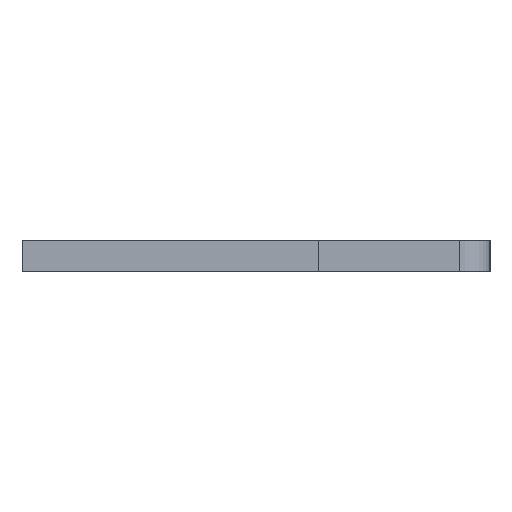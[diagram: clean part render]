
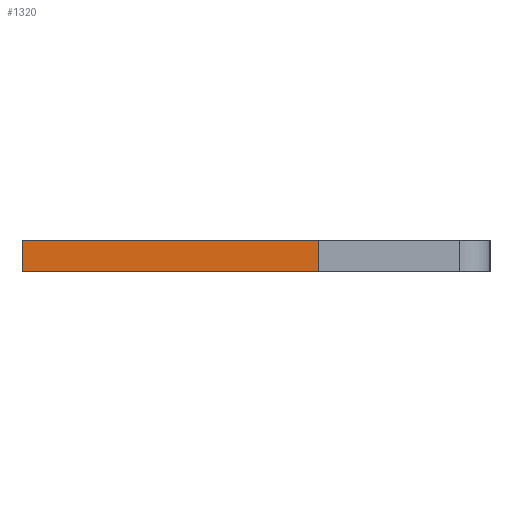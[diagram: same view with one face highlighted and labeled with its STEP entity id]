
A CAD part, left-side view. The second image highlights one B-rep face of the part: STEP entity #1320.
In plain terms, the highlighted face is planar.
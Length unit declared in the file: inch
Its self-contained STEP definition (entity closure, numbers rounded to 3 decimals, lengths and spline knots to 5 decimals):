
#26 = DIRECTION ( 'NONE',  ( -1., 0., 0. ) ) ;
#73 = EDGE_LOOP ( 'NONE', ( #1088, #316, #268, #369 ) ) ;
#86 = VECTOR ( 'NONE', #849, 39.37008 ) ;
#99 = CARTESIAN_POINT ( 'NONE',  ( 0.01, 0.15, -0.04 ) ) ;
#104 = CARTESIAN_POINT ( 'NONE',  ( 0.01, -0.04, -0.04 ) ) ;
#106 = EDGE_CURVE ( 'NONE', #1001, #947, #1057, .T. ) ;
#175 = CARTESIAN_POINT ( 'NONE',  ( -0.01, -0.04, -0.04 ) ) ;
#210 = DIRECTION ( 'NONE',  ( -1., 0., 0. ) ) ;
#268 = ORIENTED_EDGE ( 'NONE', *, *, #494, .F. ) ;
#316 = ORIENTED_EDGE ( 'NONE', *, *, #1293, .F. ) ;
#329 = CARTESIAN_POINT ( 'NONE',  ( 0.01, 0.15, -0.04 ) ) ;
#353 = VECTOR ( 'NONE', #26, 39.37008 ) ;
#369 = ORIENTED_EDGE ( 'NONE', *, *, #448, .T. ) ;
#383 = VECTOR ( 'NONE', #591, 39.37008 ) ;
#416 = CARTESIAN_POINT ( 'NONE',  ( 0.01, 0.15, -0.04 ) ) ;
#446 = FACE_OUTER_BOUND ( 'NONE', #73, .T. ) ;
#448 = EDGE_CURVE ( 'NONE', #934, #1001, #1287, .T. ) ;
#465 = CARTESIAN_POINT ( 'NONE',  ( 0.01, 0.15, -0.04 ) ) ;
#494 = EDGE_CURVE ( 'NONE', #934, #701, #1094, .T. ) ;
#528 = DIRECTION ( 'NONE',  ( 1., 0., 0. ) ) ;
#591 = DIRECTION ( 'NONE',  ( 0., 1., 0. ) ) ;
#598 = AXIS2_PLACEMENT_3D ( 'NONE', #329, #1306, #528 ) ;
#628 = VECTOR ( 'NONE', #210, 39.37008 ) ;
#642 = PLANE ( 'NONE',  #598 ) ;
#701 = VERTEX_POINT ( 'NONE', #465 ) ;
#794 = CARTESIAN_POINT ( 'NONE',  ( -0.01, 0.15, -0.04 ) ) ;
#849 = DIRECTION ( 'NONE',  ( 0., 1., 0. ) ) ;
#934 = VERTEX_POINT ( 'NONE', #1224 ) ;
#947 = VERTEX_POINT ( 'NONE', #794 ) ;
#1001 = VERTEX_POINT ( 'NONE', #175 ) ;
#1057 = LINE ( 'NONE', #1135, #383 ) ;
#1088 = ORIENTED_EDGE ( 'NONE', *, *, #106, .T. ) ;
#1094 = LINE ( 'NONE', #416, #86 ) ;
#1135 = CARTESIAN_POINT ( 'NONE',  ( -0.01, 0.15, -0.04 ) ) ;
#1224 = CARTESIAN_POINT ( 'NONE',  ( 0.01, -0.04, -0.04 ) ) ;
#1239 = LINE ( 'NONE', #99, #353 ) ;
#1287 = LINE ( 'NONE', #104, #628 ) ;
#1293 = EDGE_CURVE ( 'NONE', #701, #947, #1239, .T. ) ;
#1306 = DIRECTION ( 'NONE',  ( 0., 0., 1. ) ) ;
#1320 = ADVANCED_FACE ( 'NONE', ( #446 ), #642, .F. ) ;
